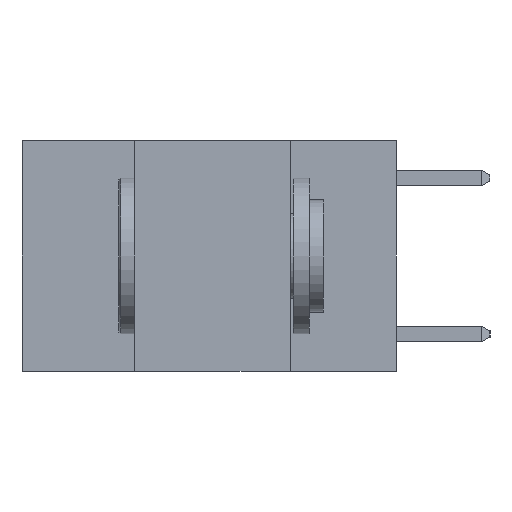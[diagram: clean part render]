
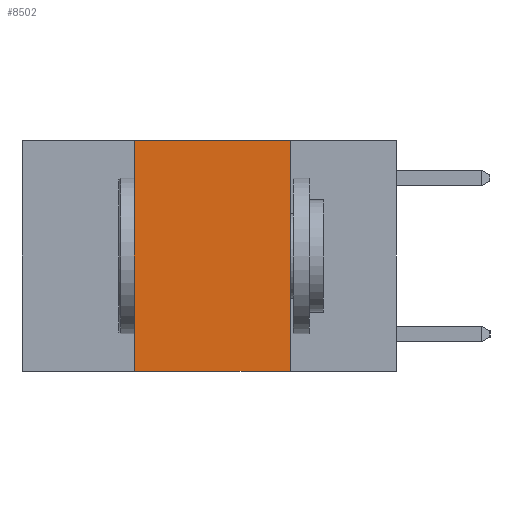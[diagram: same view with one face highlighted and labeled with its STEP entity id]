
A CAD part, left-side view. The second image highlights one B-rep face of the part: STEP entity #8502.
In plain terms, the highlighted planar face has unit normal (-1, 0, 0).
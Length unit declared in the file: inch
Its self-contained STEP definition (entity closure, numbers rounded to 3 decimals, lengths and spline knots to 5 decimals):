
#181 = EDGE_CURVE ( 'NONE', #3640, #3840, #8458, .T. ) ;
#537 = VECTOR ( 'NONE', #1300, 39.37008 ) ;
#823 = CARTESIAN_POINT ( 'NONE',  ( 0., 0.17, 0. ) ) ;
#938 = VECTOR ( 'NONE', #7209, 39.37008 ) ;
#1300 = DIRECTION ( 'NONE',  ( 0., -1., 0. ) ) ;
#1419 = PLANE ( 'NONE',  #4644 ) ;
#1505 = ORIENTED_EDGE ( 'NONE', *, *, #181, .F. ) ;
#2166 = DIRECTION ( 'NONE',  ( 1., 0., 0. ) ) ;
#2534 = VECTOR ( 'NONE', #9022, 39.37008 ) ;
#2545 = LINE ( 'NONE', #5682, #537 ) ;
#2653 = DIRECTION ( 'NONE',  ( 0., 0., 1. ) ) ;
#3134 = VERTEX_POINT ( 'NONE', #4379 ) ;
#3640 = VERTEX_POINT ( 'NONE', #5360 ) ;
#3840 = VERTEX_POINT ( 'NONE', #823 ) ;
#4379 = CARTESIAN_POINT ( 'NONE',  ( 0., 0.17, -0.37 ) ) ;
#4644 = AXIS2_PLACEMENT_3D ( 'NONE', #6531, #2166, #7267 ) ;
#4814 = CARTESIAN_POINT ( 'NONE',  ( 0., 0.42, 0. ) ) ;
#5192 = ORIENTED_EDGE ( 'NONE', *, *, #9006, .T. ) ;
#5360 = CARTESIAN_POINT ( 'NONE',  ( 0., 0.42, 0. ) ) ;
#5661 = ORIENTED_EDGE ( 'NONE', *, *, #7769, .F. ) ;
#5682 = CARTESIAN_POINT ( 'NONE',  ( 0., 0.6, -0.37 ) ) ;
#5971 = VECTOR ( 'NONE', #2653, 39.37008 ) ;
#5991 = VERTEX_POINT ( 'NONE', #9197 ) ;
#6383 = LINE ( 'NONE', #7585, #2534 ) ;
#6531 = CARTESIAN_POINT ( 'NONE',  ( 0., 0.6, 0. ) ) ;
#7209 = DIRECTION ( 'NONE',  ( 0., -1., 0. ) ) ;
#7232 = CARTESIAN_POINT ( 'NONE',  ( 0., 0.6, 0. ) ) ;
#7267 = DIRECTION ( 'NONE',  ( 0., 0., -1. ) ) ;
#7501 = ORIENTED_EDGE ( 'NONE', *, *, #9395, .F. ) ;
#7557 = FACE_OUTER_BOUND ( 'NONE', #9425, .T. ) ;
#7585 = CARTESIAN_POINT ( 'NONE',  ( 0., 0.17, 0. ) ) ;
#7769 = EDGE_CURVE ( 'NONE', #5991, #3640, #7902, .T. ) ;
#7902 = LINE ( 'NONE', #4814, #5971 ) ;
#8458 = LINE ( 'NONE', #7232, #938 ) ;
#8502 = ADVANCED_FACE ( 'NONE', ( #7557 ), #1419, .F. ) ;
#9006 = EDGE_CURVE ( 'NONE', #5991, #3134, #2545, .T. ) ;
#9022 = DIRECTION ( 'NONE',  ( 0., 0., -1. ) ) ;
#9197 = CARTESIAN_POINT ( 'NONE',  ( 0., 0.42, -0.37 ) ) ;
#9395 = EDGE_CURVE ( 'NONE', #3840, #3134, #6383, .T. ) ;
#9425 = EDGE_LOOP ( 'NONE', ( #7501, #1505, #5661, #5192 ) ) ;
